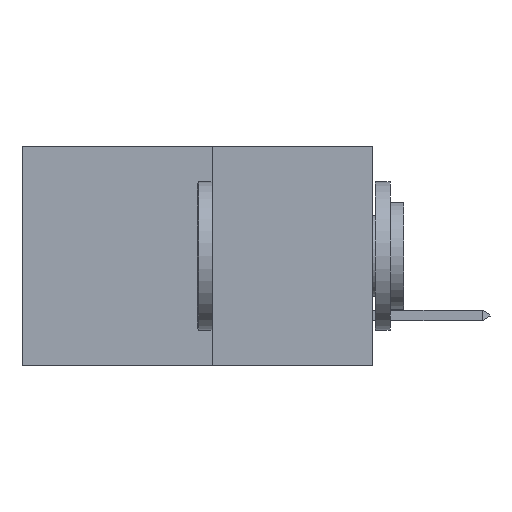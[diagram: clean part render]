
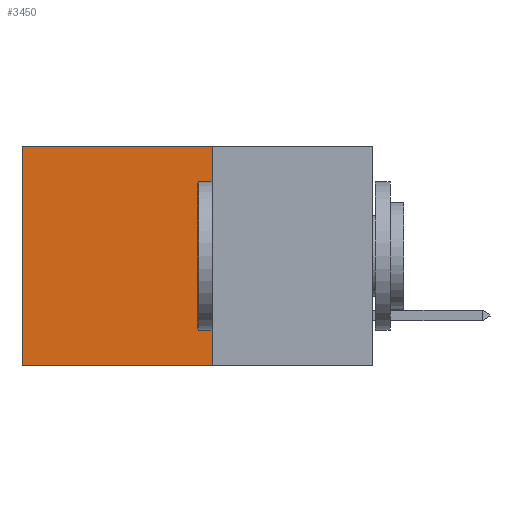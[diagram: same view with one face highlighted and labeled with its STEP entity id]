
A CAD part, left-side view. The second image highlights one B-rep face of the part: STEP entity #3450.
In plain terms, the highlighted planar face has unit normal (-1, 0, 0).
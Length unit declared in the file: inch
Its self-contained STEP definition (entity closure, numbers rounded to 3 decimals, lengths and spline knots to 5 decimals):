
#422 = CARTESIAN_POINT ( 'NONE',  ( 0.277, 0.27, -0.37 ) ) ;
#899 = LINE ( 'NONE', #12793, #9994 ) ;
#1235 = VECTOR ( 'NONE', #5145, 39.37008 ) ;
#1520 = CARTESIAN_POINT ( 'NONE',  ( 0.277, 0.59, -0.37 ) ) ;
#1655 = AXIS2_PLACEMENT_3D ( 'NONE', #10587, #10572, #10523 ) ;
#1906 = VERTEX_POINT ( 'NONE', #11692 ) ;
#2123 = VECTOR ( 'NONE', #7972, 39.37008 ) ;
#2741 = DIRECTION ( 'NONE',  ( 0., 1., 0. ) ) ;
#3450 = ADVANCED_FACE ( 'NONE', ( #13263 ), #10620, .F. ) ;
#3679 = LINE ( 'NONE', #14867, #6450 ) ;
#3738 = VERTEX_POINT ( 'NONE', #7318 ) ;
#4849 = VERTEX_POINT ( 'NONE', #1520 ) ;
#4963 = EDGE_CURVE ( 'NONE', #3738, #4849, #3679, .T. ) ;
#5145 = DIRECTION ( 'NONE',  ( 0., 0., -1. ) ) ;
#5304 = LINE ( 'NONE', #13669, #2123 ) ;
#5622 = ORIENTED_EDGE ( 'NONE', *, *, #4963, .F. ) ;
#6450 = VECTOR ( 'NONE', #2741, 39.37008 ) ;
#6680 = CARTESIAN_POINT ( 'NONE',  ( 0.277, 0.59, 0. ) ) ;
#6841 = EDGE_CURVE ( 'NONE', #1906, #10513, #5304, .T. ) ;
#7318 = CARTESIAN_POINT ( 'NONE',  ( 0.277, 0.27, -0.37 ) ) ;
#7972 = DIRECTION ( 'NONE',  ( 0., 1., 0. ) ) ;
#8226 = EDGE_CURVE ( 'NONE', #10513, #4849, #899, .T. ) ;
#9092 = EDGE_CURVE ( 'NONE', #1906, #3738, #13656, .T. ) ;
#9994 = VECTOR ( 'NONE', #13899, 39.37008 ) ;
#10513 = VERTEX_POINT ( 'NONE', #6680 ) ;
#10523 = DIRECTION ( 'NONE',  ( 0., 0., -1. ) ) ;
#10572 = DIRECTION ( 'NONE',  ( 1., 0., 0. ) ) ;
#10587 = CARTESIAN_POINT ( 'NONE',  ( 0.277, 0.27, -0.37 ) ) ;
#10620 = PLANE ( 'NONE',  #1655 ) ;
#11692 = CARTESIAN_POINT ( 'NONE',  ( 0.277, 0.27, 0. ) ) ;
#12395 = EDGE_LOOP ( 'NONE', ( #13214, #5622, #12527, #13940 ) ) ;
#12527 = ORIENTED_EDGE ( 'NONE', *, *, #9092, .F. ) ;
#12793 = CARTESIAN_POINT ( 'NONE',  ( 0.277, 0.59, -0.37 ) ) ;
#13214 = ORIENTED_EDGE ( 'NONE', *, *, #8226, .T. ) ;
#13263 = FACE_OUTER_BOUND ( 'NONE', #12395, .T. ) ;
#13656 = LINE ( 'NONE', #422, #1235 ) ;
#13669 = CARTESIAN_POINT ( 'NONE',  ( 0.277, 0.27, 0. ) ) ;
#13899 = DIRECTION ( 'NONE',  ( 0., 0., -1. ) ) ;
#13940 = ORIENTED_EDGE ( 'NONE', *, *, #6841, .T. ) ;
#14867 = CARTESIAN_POINT ( 'NONE',  ( 0.277, 0.27, -0.37 ) ) ;
